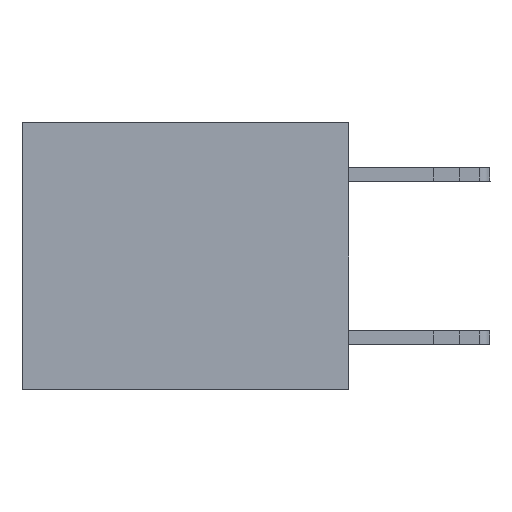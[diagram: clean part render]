
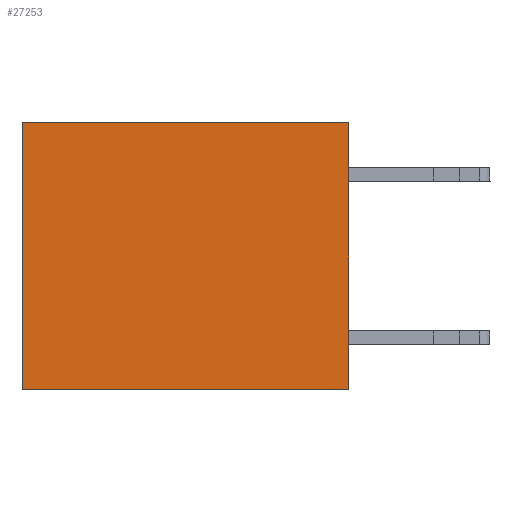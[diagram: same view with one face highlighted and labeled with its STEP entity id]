
A CAD part, left-side view. The second image highlights one B-rep face of the part: STEP entity #27253.
In plain terms, the highlighted planar face has unit normal (-1, 0, 0).
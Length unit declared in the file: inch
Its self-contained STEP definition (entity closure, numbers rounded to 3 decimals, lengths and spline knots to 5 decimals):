
#937 = DIRECTION ( 'NONE',  ( 0., 0., -1. ) ) ;
#2631 = CARTESIAN_POINT ( 'NONE',  ( 0.3165, 0., -0.49 ) ) ;
#3069 = VECTOR ( 'NONE', #15407, 39.37008 ) ;
#3662 = AXIS2_PLACEMENT_3D ( 'NONE', #13384, #30624, #20826 ) ;
#3682 = DIRECTION ( 'NONE',  ( 0., 0., -1. ) ) ;
#3955 = EDGE_CURVE ( 'NONE', #23995, #24929, #23696, .T. ) ;
#3999 = EDGE_LOOP ( 'NONE', ( #14075, #4830, #22493, #22801 ) ) ;
#4376 = VERTEX_POINT ( 'NONE', #6608 ) ;
#4830 = ORIENTED_EDGE ( 'NONE', *, *, #24301, .F. ) ;
#5099 = CARTESIAN_POINT ( 'NONE',  ( 0.3165, 0.6, -0.49 ) ) ;
#6608 = CARTESIAN_POINT ( 'NONE',  ( 0.3165, 0., -0.49 ) ) ;
#6736 = FACE_OUTER_BOUND ( 'NONE', #3999, .T. ) ;
#6878 = LINE ( 'NONE', #12412, #3069 ) ;
#10726 = VERTEX_POINT ( 'NONE', #17922 ) ;
#11227 = CARTESIAN_POINT ( 'NONE',  ( 0.3165, 0.6, 0. ) ) ;
#12412 = CARTESIAN_POINT ( 'NONE',  ( 0.3165, 0., -0.49 ) ) ;
#13384 = CARTESIAN_POINT ( 'NONE',  ( 0.3165, 0., -0.49 ) ) ;
#14075 = ORIENTED_EDGE ( 'NONE', *, *, #3955, .T. ) ;
#14439 = LINE ( 'NONE', #15102, #30244 ) ;
#14794 = VECTOR ( 'NONE', #3682, 39.37008 ) ;
#15102 = CARTESIAN_POINT ( 'NONE',  ( 0.3165, 0., 0. ) ) ;
#15407 = DIRECTION ( 'NONE',  ( 0., 1., 0. ) ) ;
#15459 = EDGE_CURVE ( 'NONE', #10726, #23995, #14439, .T. ) ;
#17149 = VECTOR ( 'NONE', #937, 39.37008 ) ;
#17744 = CARTESIAN_POINT ( 'NONE',  ( 0.3165, 0.6, -0.49 ) ) ;
#17922 = CARTESIAN_POINT ( 'NONE',  ( 0.3165, 0., 0. ) ) ;
#20826 = DIRECTION ( 'NONE',  ( 0., 0., -1. ) ) ;
#22493 = ORIENTED_EDGE ( 'NONE', *, *, #26655, .F. ) ;
#22801 = ORIENTED_EDGE ( 'NONE', *, *, #15459, .T. ) ;
#23696 = LINE ( 'NONE', #5099, #17149 ) ;
#23995 = VERTEX_POINT ( 'NONE', #11227 ) ;
#24301 = EDGE_CURVE ( 'NONE', #4376, #24929, #6878, .T. ) ;
#24929 = VERTEX_POINT ( 'NONE', #17744 ) ;
#25346 = DIRECTION ( 'NONE',  ( 0., 1., 0. ) ) ;
#26655 = EDGE_CURVE ( 'NONE', #10726, #4376, #27901, .T. ) ;
#27253 = ADVANCED_FACE ( 'NONE', ( #6736 ), #28131, .F. ) ;
#27901 = LINE ( 'NONE', #2631, #14794 ) ;
#28131 = PLANE ( 'NONE',  #3662 ) ;
#30244 = VECTOR ( 'NONE', #25346, 39.37008 ) ;
#30624 = DIRECTION ( 'NONE',  ( 1., 0., 0. ) ) ;
